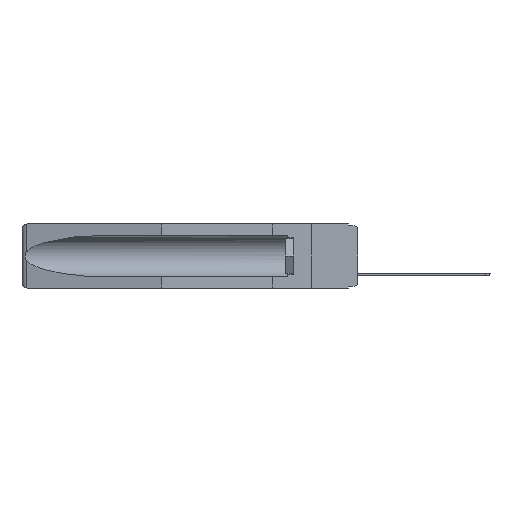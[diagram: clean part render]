
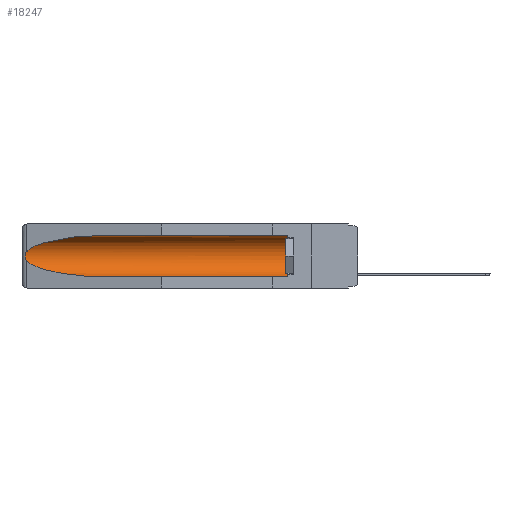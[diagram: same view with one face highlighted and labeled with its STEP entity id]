
A CAD part, left-side view. The second image highlights one B-rep face of the part: STEP entity #18247.
In plain terms, the highlighted cylindrical face has radius 2.857 mm (diameter 5.715 mm), a partial arc.
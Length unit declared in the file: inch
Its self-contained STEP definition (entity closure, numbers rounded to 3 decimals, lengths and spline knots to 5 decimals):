
#119 = VERTEX_POINT ( 'NONE', #1852 ) ;
#201 = EDGE_CURVE ( 'NONE', #21741, #26842, #26122, .T. ) ;
#221 = CARTESIAN_POINT ( 'NONE',  ( 0.26537, 1.52718, -0.14972 ) ) ;
#1423 = CARTESIAN_POINT ( 'NONE',  ( 0.155, 0.126, -0.059 ) ) ;
#1849 = CARTESIAN_POINT ( 'NONE',  ( 0.155, 1.07973, -0.284 ) ) ;
#1852 = CARTESIAN_POINT ( 'NONE',  ( 0.155, 1.07973, -0.059 ) ) ;
#2431 = B_SPLINE_CURVE_WITH_KNOTS ( 'NONE', 3,
 ( #7747, #3159, #13886, #22518, #9640, #26614, #24424, #15883, #7655, #22336 ),
 .UNSPECIFIED., .F., .F.,
 ( 4, 2, 2, 2, 4 ),
 ( 0., 0.00029, 0.00058, 0.00087, 0.00117 ),
 .UNSPECIFIED. ) ;
#3159 = CARTESIAN_POINT ( 'NONE',  ( 0.26597, 1.52961, -0.15275 ) ) ;
#3764 = CARTESIAN_POINT ( 'NONE',  ( 0.21114, 1.30732, -0.059 ) ) ;
#3833 = CARTESIAN_POINT ( 'NONE',  ( 0.155, 0.126, -0.284 ) ) ;
#3980 = CARTESIAN_POINT ( 'NONE',  ( 0.25451, 1.48313, -0.24835 ) ) ;
#4452 = EDGE_CURVE ( 'NONE', #119, #12421, #14882, .T. ) ;
#5720 = EDGE_CURVE ( 'NONE', #21741, #23108, #23464, .T. ) ;
#5814 = CARTESIAN_POINT ( 'NONE',  ( 0.155, -0.30754, -0.284 ) ) ;
#5830 = CARTESIAN_POINT ( 'NONE',  ( 0.155, 1.07973, -0.059 ) ) ;
#5860 = DIRECTION ( 'NONE',  ( 0., 1., 0. ) ) ;
#5934 = CARTESIAN_POINT ( 'NONE',  ( 0.26537, 1.52718, -0.19328 ) ) ;
#6489 = AXIS2_PLACEMENT_3D ( 'NONE', #14325, #5860, #18531 ) ;
#7471 = DIRECTION ( 'NONE',  ( 0., -1., 0. ) ) ;
#7655 = CARTESIAN_POINT ( 'NONE',  ( 0.26597, 1.5296, -0.19026 ) ) ;
#7747 = CARTESIAN_POINT ( 'NONE',  ( 0.26537, 1.52718, -0.14972 ) ) ;
#8773 = EDGE_CURVE ( 'NONE', #23108, #119, #11538, .T. ) ;
#8788 = CARTESIAN_POINT ( 'NONE',  ( 0.155, 1.07973, -0.284 ) ) ;
#9221 = DIRECTION ( 'NONE',  ( 0., 0., 1. ) ) ;
#9509 = AXIS2_PLACEMENT_3D ( 'NONE', #20141, #7471, #9221 ) ;
#9640 = CARTESIAN_POINT ( 'NONE',  ( 0.2675, 1.53308, -0.16763 ) ) ;
#9788 = CARTESIAN_POINT ( 'NONE',  ( 0.25451, 1.48313, -0.09465 ) ) ;
#10003 = CARTESIAN_POINT ( 'NONE',  ( 0.21114, 1.30732, -0.284 ) ) ;
#11538 = LINE ( 'NONE', #23980, #17078 ) ;
#11973 = EDGE_LOOP ( 'NONE', ( #26909, #18568, #17041, #23454, #24531, #13776 ) ) ;
#12421 = VERTEX_POINT ( 'NONE', #221 ) ;
#13776 = ORIENTED_EDGE ( 'NONE', *, *, #8773, .T. ) ;
#13886 = CARTESIAN_POINT ( 'NONE',  ( 0.26654, 1.53092, -0.15636 ) ) ;
#14325 = CARTESIAN_POINT ( 'NONE',  ( 0.155, -0.30754, -0.1715 ) ) ;
#14882 =( BOUNDED_CURVE ( )  B_SPLINE_CURVE ( 3, ( #5830, #3764, #9788, #22661 ),
 .UNSPECIFIED., .F., .F. ) 
 B_SPLINE_CURVE_WITH_KNOTS ( ( 4, 4 ),
 ( 4.71239, 6.08839 ),
 .UNSPECIFIED. ) 
 CURVE ( )  GEOMETRIC_REPRESENTATION_ITEM ( )  RATIONAL_B_SPLINE_CURVE ( ( 1., 0.848, 0.848, 1. ) ) 
 REPRESENTATION_ITEM ( '' )  );
#15883 = CARTESIAN_POINT ( 'NONE',  ( 0.26655, 1.53094, -0.18657 ) ) ;
#16349 = CARTESIAN_POINT ( 'NONE',  ( 0.26537, 1.52718, -0.19328 ) ) ;
#17041 = ORIENTED_EDGE ( 'NONE', *, *, #22293, .T. ) ;
#17078 = VECTOR ( 'NONE', #22275, 39.37008 ) ;
#18247 = ADVANCED_FACE ( 'NONE', ( #21140 ), #21471, .F. ) ;
#18531 = DIRECTION ( 'NONE',  ( 0., 0., 1. ) ) ;
#18568 = ORIENTED_EDGE ( 'NONE', *, *, #22171, .T. ) ;
#20141 = CARTESIAN_POINT ( 'NONE',  ( 0.155, 0.126, -0.1715 ) ) ;
#20630 =( BOUNDED_CURVE ( )  B_SPLINE_CURVE ( 3, ( #16349, #3980, #10003, #1849 ),
 .UNSPECIFIED., .F., .T. ) 
 B_SPLINE_CURVE_WITH_KNOTS ( ( 4, 4 ),
 ( 0.1948, 1.5708 ),
 .UNSPECIFIED. ) 
 CURVE ( )  GEOMETRIC_REPRESENTATION_ITEM ( )  RATIONAL_B_SPLINE_CURVE ( ( 1., 0.848, 0.848, 1. ) ) 
 REPRESENTATION_ITEM ( '' )  );
#21140 = FACE_OUTER_BOUND ( 'NONE', #11973, .T. ) ;
#21471 = CYLINDRICAL_SURFACE ( 'NONE', #6489, 0.1125 ) ;
#21741 = VERTEX_POINT ( 'NONE', #3833 ) ;
#22171 = EDGE_CURVE ( 'NONE', #12421, #24577, #2431, .T. ) ;
#22275 = DIRECTION ( 'NONE',  ( 0., 1., 0. ) ) ;
#22293 = EDGE_CURVE ( 'NONE', #24577, #26842, #20630, .T. ) ;
#22336 = CARTESIAN_POINT ( 'NONE',  ( 0.26537, 1.52718, -0.19328 ) ) ;
#22518 = CARTESIAN_POINT ( 'NONE',  ( 0.2673, 1.5327, -0.16383 ) ) ;
#22661 = CARTESIAN_POINT ( 'NONE',  ( 0.26537, 1.52718, -0.14972 ) ) ;
#23108 = VERTEX_POINT ( 'NONE', #1423 ) ;
#23174 = VECTOR ( 'NONE', #24913, 39.37008 ) ;
#23454 = ORIENTED_EDGE ( 'NONE', *, *, #201, .F. ) ;
#23464 = CIRCLE ( 'NONE', #9509, 0.1125 ) ;
#23980 = CARTESIAN_POINT ( 'NONE',  ( 0.155, -0.30754, -0.059 ) ) ;
#24424 = CARTESIAN_POINT ( 'NONE',  ( 0.2673, 1.53269, -0.17917 ) ) ;
#24531 = ORIENTED_EDGE ( 'NONE', *, *, #5720, .T. ) ;
#24577 = VERTEX_POINT ( 'NONE', #5934 ) ;
#24913 = DIRECTION ( 'NONE',  ( 0., 1., 0. ) ) ;
#26122 = LINE ( 'NONE', #5814, #23174 ) ;
#26614 = CARTESIAN_POINT ( 'NONE',  ( 0.2675, 1.53308, -0.17534 ) ) ;
#26842 = VERTEX_POINT ( 'NONE', #8788 ) ;
#26909 = ORIENTED_EDGE ( 'NONE', *, *, #4452, .T. ) ;
